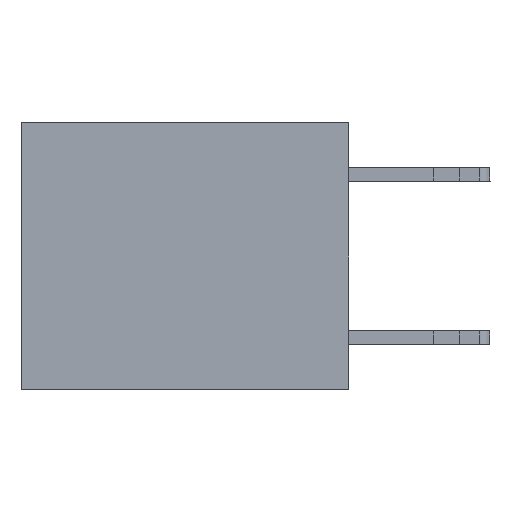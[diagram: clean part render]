
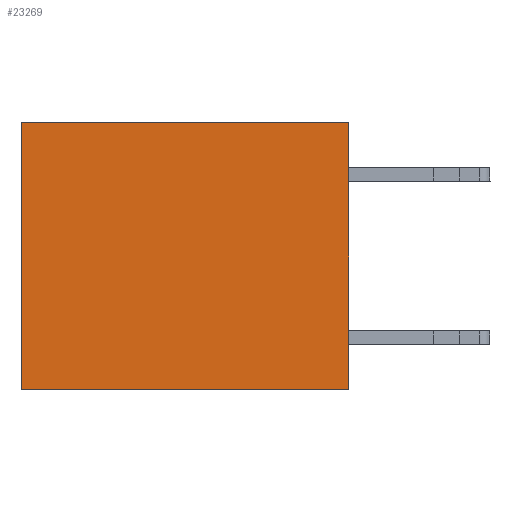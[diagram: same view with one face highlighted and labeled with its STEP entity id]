
A CAD part, left-side view. The second image highlights one B-rep face of the part: STEP entity #23269.
In plain terms, the highlighted planar face has unit normal (-1, 0, 0).
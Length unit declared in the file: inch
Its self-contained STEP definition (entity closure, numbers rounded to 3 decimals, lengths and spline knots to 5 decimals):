
#823 = AXIS2_PLACEMENT_3D ( 'NONE', #15242, #17547, #15726 ) ;
#845 = VECTOR ( 'NONE', #14781, 39.37008 ) ;
#865 = CARTESIAN_POINT ( 'NONE',  ( 0.3165, 0.6, -0.49 ) ) ;
#897 = LINE ( 'NONE', #13452, #22780 ) ;
#2142 = CARTESIAN_POINT ( 'NONE',  ( 0.3165, 0., -0.49 ) ) ;
#5188 = EDGE_CURVE ( 'NONE', #14771, #9572, #19845, .T. ) ;
#5200 = LINE ( 'NONE', #18502, #845 ) ;
#5609 = LINE ( 'NONE', #2142, #15823 ) ;
#8040 = PLANE ( 'NONE',  #823 ) ;
#8503 = FACE_OUTER_BOUND ( 'NONE', #19167, .T. ) ;
#9572 = VERTEX_POINT ( 'NONE', #21251 ) ;
#10050 = ORIENTED_EDGE ( 'NONE', *, *, #15318, .F. ) ;
#11011 = EDGE_CURVE ( 'NONE', #22765, #12626, #5200, .T. ) ;
#11653 = DIRECTION ( 'NONE',  ( 0., 1., 0. ) ) ;
#11788 = CARTESIAN_POINT ( 'NONE',  ( 0.3165, 0.6, 0. ) ) ;
#12626 = VERTEX_POINT ( 'NONE', #22464 ) ;
#13452 = CARTESIAN_POINT ( 'NONE',  ( 0.3165, 0., 0. ) ) ;
#13815 = CARTESIAN_POINT ( 'NONE',  ( 0.3165, 0., 0. ) ) ;
#14575 = VECTOR ( 'NONE', #17693, 39.37008 ) ;
#14771 = VERTEX_POINT ( 'NONE', #11788 ) ;
#14781 = DIRECTION ( 'NONE',  ( 0., 0., -1. ) ) ;
#15242 = CARTESIAN_POINT ( 'NONE',  ( 0.3165, 0., -0.49 ) ) ;
#15318 = EDGE_CURVE ( 'NONE', #12626, #9572, #5609, .T. ) ;
#15726 = DIRECTION ( 'NONE',  ( 0., 0., -1. ) ) ;
#15822 = ORIENTED_EDGE ( 'NONE', *, *, #11011, .F. ) ;
#15823 = VECTOR ( 'NONE', #17064, 39.37008 ) ;
#16177 = EDGE_CURVE ( 'NONE', #22765, #14771, #897, .T. ) ;
#16813 = ORIENTED_EDGE ( 'NONE', *, *, #5188, .T. ) ;
#17064 = DIRECTION ( 'NONE',  ( 0., 1., 0. ) ) ;
#17547 = DIRECTION ( 'NONE',  ( 1., 0., 0. ) ) ;
#17693 = DIRECTION ( 'NONE',  ( 0., 0., -1. ) ) ;
#17873 = ORIENTED_EDGE ( 'NONE', *, *, #16177, .T. ) ;
#18502 = CARTESIAN_POINT ( 'NONE',  ( 0.3165, 0., -0.49 ) ) ;
#19167 = EDGE_LOOP ( 'NONE', ( #16813, #10050, #15822, #17873 ) ) ;
#19845 = LINE ( 'NONE', #865, #14575 ) ;
#21251 = CARTESIAN_POINT ( 'NONE',  ( 0.3165, 0.6, -0.49 ) ) ;
#22464 = CARTESIAN_POINT ( 'NONE',  ( 0.3165, 0., -0.49 ) ) ;
#22765 = VERTEX_POINT ( 'NONE', #13815 ) ;
#22780 = VECTOR ( 'NONE', #11653, 39.37008 ) ;
#23269 = ADVANCED_FACE ( 'NONE', ( #8503 ), #8040, .F. ) ;
